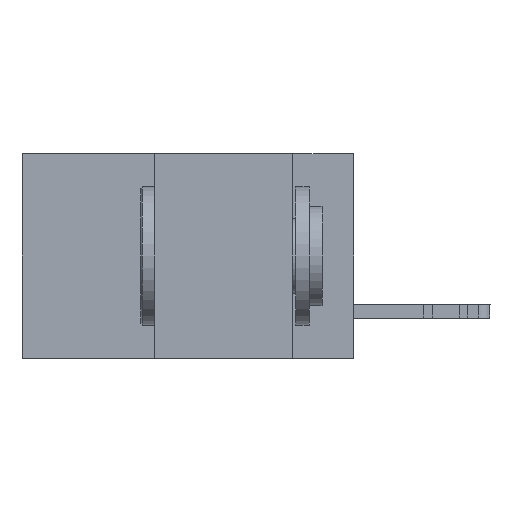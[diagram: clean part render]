
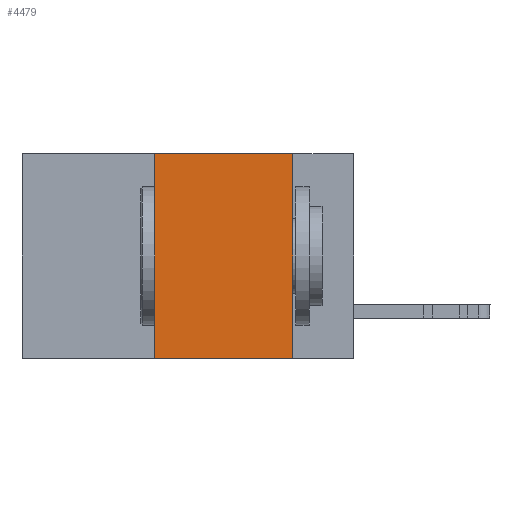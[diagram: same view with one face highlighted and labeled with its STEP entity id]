
A CAD part, left-side view. The second image highlights one B-rep face of the part: STEP entity #4479.
In plain terms, the highlighted planar face has unit normal (-1, 0, 0).
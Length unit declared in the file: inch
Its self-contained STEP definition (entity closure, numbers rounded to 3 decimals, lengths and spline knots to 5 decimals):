
#2665 = CARTESIAN_POINT ( 'NONE',  ( 0., 0.6, 0. ) ) ;
#3247 = VECTOR ( 'NONE', #19028, 39.37008 ) ;
#4111 = VECTOR ( 'NONE', #29209, 39.37008 ) ;
#4479 = ADVANCED_FACE ( 'NONE', ( #45529 ), #17273, .F. ) ;
#5976 = DIRECTION ( 'NONE',  ( 0., 0., 1. ) ) ;
#8590 = ORIENTED_EDGE ( 'NONE', *, *, #41316, .T. ) ;
#8648 = LINE ( 'NONE', #26084, #3247 ) ;
#10650 = VECTOR ( 'NONE', #5976, 39.37008 ) ;
#10816 = ORIENTED_EDGE ( 'NONE', *, *, #45133, .F. ) ;
#11189 = DIRECTION ( 'NONE',  ( 0., -1., 0. ) ) ;
#12334 = EDGE_CURVE ( 'NONE', #21046, #16430, #24093, .T. ) ;
#12734 = CARTESIAN_POINT ( 'NONE',  ( 0., 0.36, -0.37 ) ) ;
#13266 = DIRECTION ( 'NONE',  ( 0., 0., -1. ) ) ;
#14717 = ORIENTED_EDGE ( 'NONE', *, *, #12334, .F. ) ;
#14855 = LINE ( 'NONE', #36746, #4111 ) ;
#16430 = VERTEX_POINT ( 'NONE', #32495 ) ;
#17273 = PLANE ( 'NONE',  #44214 ) ;
#18788 = CARTESIAN_POINT ( 'NONE',  ( 0., 0.11, 0. ) ) ;
#19028 = DIRECTION ( 'NONE',  ( 0., -1., 0. ) ) ;
#19850 = VERTEX_POINT ( 'NONE', #41693 ) ;
#21046 = VERTEX_POINT ( 'NONE', #12734 ) ;
#23628 = DIRECTION ( 'NONE',  ( 1., 0., 0. ) ) ;
#24014 = VERTEX_POINT ( 'NONE', #18788 ) ;
#24093 = LINE ( 'NONE', #24324, #10650 ) ;
#24324 = CARTESIAN_POINT ( 'NONE',  ( 0., 0.36, 0. ) ) ;
#26084 = CARTESIAN_POINT ( 'NONE',  ( 0., 0.6, -0.37 ) ) ;
#28274 = ORIENTED_EDGE ( 'NONE', *, *, #34310, .F. ) ;
#29093 = LINE ( 'NONE', #43452, #42990 ) ;
#29209 = DIRECTION ( 'NONE',  ( 0., 0., -1. ) ) ;
#32495 = CARTESIAN_POINT ( 'NONE',  ( 0., 0.36, 0. ) ) ;
#32987 = EDGE_LOOP ( 'NONE', ( #10816, #28274, #14717, #8590 ) ) ;
#34310 = EDGE_CURVE ( 'NONE', #16430, #24014, #29093, .T. ) ;
#36746 = CARTESIAN_POINT ( 'NONE',  ( 0., 0.11, 0. ) ) ;
#41316 = EDGE_CURVE ( 'NONE', #21046, #19850, #8648, .T. ) ;
#41693 = CARTESIAN_POINT ( 'NONE',  ( 0., 0.11, -0.37 ) ) ;
#42990 = VECTOR ( 'NONE', #11189, 39.37008 ) ;
#43452 = CARTESIAN_POINT ( 'NONE',  ( 0., 0.6, 0. ) ) ;
#44214 = AXIS2_PLACEMENT_3D ( 'NONE', #2665, #23628, #13266 ) ;
#45133 = EDGE_CURVE ( 'NONE', #24014, #19850, #14855, .T. ) ;
#45529 = FACE_OUTER_BOUND ( 'NONE', #32987, .T. ) ;
